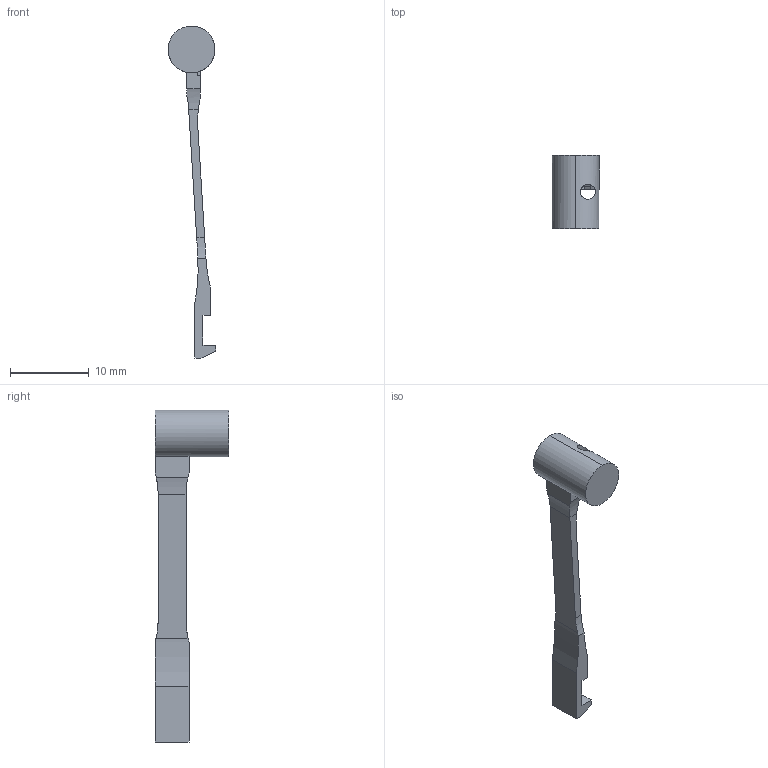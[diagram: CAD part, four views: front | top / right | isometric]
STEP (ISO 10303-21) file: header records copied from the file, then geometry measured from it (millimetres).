
FILE_DESCRIPTION (( 'STEP AP214' ), '1' );
FILE_NAME ('EXTRACTOR - XD-40 TACTICAL.STEP', '2013-06-19T14:02:27', ( 'Asher' ), ( '' ), 'SwSTEP 2.0', 'SolidWorks 2013', '' );
FILE_SCHEMA (( 'AUTOMOTIVE_DESIGN' ));
Length unit declared in the file: millimetre
Products named in the file (1): EXTRACTOR - XD-40 TACTICAL
Bounding box: 6.1 x 9.4 x 42.29 mm (x, y, z)
Volume: 432.6 mm3; surface area: 644.4 mm2
Topology: 1 solids, 1 shells, 32 faces, 93 edges, 62 vertices
Faces by surface type: plane 20, cylinder 12
Entity records: 1161 total; most frequent: CARTESIAN_POINT 289, ORIENTED_EDGE 186, DIRECTION 163, EDGE_CURVE 93, VERTEX_POINT 62, LINE 59, VECTOR 59, AXIS2_PLACEMENT_3D 52
